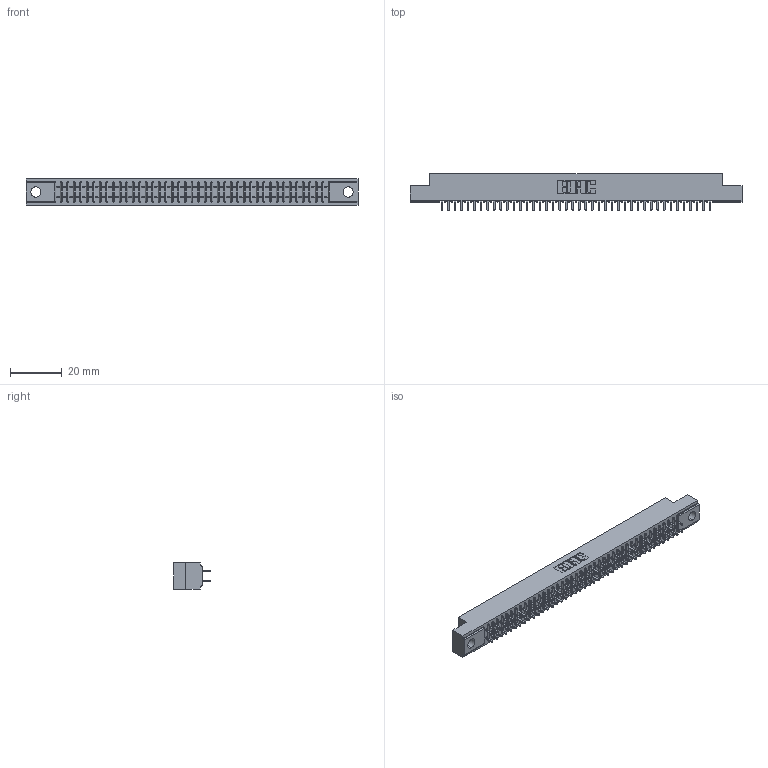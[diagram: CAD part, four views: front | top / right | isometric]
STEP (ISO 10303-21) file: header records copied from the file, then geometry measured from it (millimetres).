
FILE_DESCRIPTION (( 'STEP AP203' ), '1' );
FILE_NAME ('391-084-520-204.STEP', '2018-08-09T16:14:23', ( '' ), ( '' ), 'SwSTEP 2.0', 'SolidWorks 2016', '' );
FILE_SCHEMA (( 'CONFIG_CONTROL_DESIGN' ));
Length unit declared in the file: inch
Products named in the file (3): 341 Part_.156 (3.96) Dia Mounting Holes; 341-292-001_341-292-120; 391-084-520-204
Assembly tree (85 placements, depth 2):
  391-084-520-204
    341 Part_.156 (3.96) Dia Mounting Holes
    341-292-001_341-292-120  x84
Bounding box: 128.91 x 14.27 x 10.16 mm (x, y, z)
Volume: 9416.3 mm3; surface area: 16522.7 mm2
Topology: 85 solids, 85 shells, 5674 faces, 16438 edges, 10646 vertices
Faces by surface type: plane 3442, cylinder 2064, sphere 86, torus 82
Entity records: 51247 total; most frequent: CARTESIAN_POINT 8524, ORIENTED_EDGE 8468, DIRECTION 8264, EDGE_CURVE 4234, LINE 3428, VECTOR 3428, VERTEX_POINT 2678, AXIS2_PLACEMENT_3D 2418
